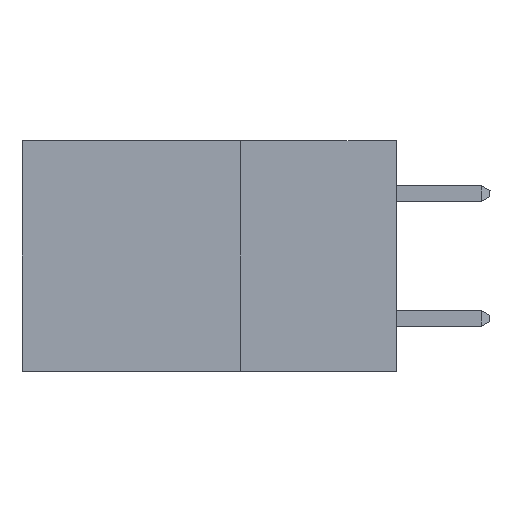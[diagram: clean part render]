
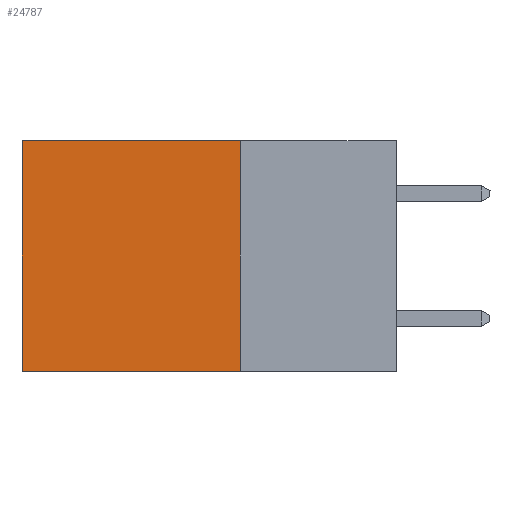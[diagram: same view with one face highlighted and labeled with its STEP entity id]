
A CAD part, left-side view. The second image highlights one B-rep face of the part: STEP entity #24787.
In plain terms, the highlighted planar face has unit normal (-1, 0, 0).
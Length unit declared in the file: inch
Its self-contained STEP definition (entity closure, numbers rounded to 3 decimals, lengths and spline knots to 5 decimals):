
#172 = CARTESIAN_POINT ( 'NONE',  ( 0.298, 0.6, 0. ) ) ;
#449 = VECTOR ( 'NONE', #8742, 39.37008 ) ;
#776 = LINE ( 'NONE', #6904, #15609 ) ;
#1443 = LINE ( 'NONE', #18984, #12046 ) ;
#1630 = ORIENTED_EDGE ( 'NONE', *, *, #18000, .F. ) ;
#1728 = EDGE_CURVE ( 'NONE', #15118, #23663, #1443, .T. ) ;
#1794 = CARTESIAN_POINT ( 'NONE',  ( 0.298, 0.25, -0.37 ) ) ;
#2021 = EDGE_CURVE ( 'NONE', #23663, #22549, #16575, .T. ) ;
#3612 = PLANE ( 'NONE',  #17691 ) ;
#5741 = DIRECTION ( 'NONE',  ( 0., 0., -1. ) ) ;
#6333 = ORIENTED_EDGE ( 'NONE', *, *, #1728, .T. ) ;
#6855 = CARTESIAN_POINT ( 'NONE',  ( 0.298, 0.25, -0.37 ) ) ;
#6904 = CARTESIAN_POINT ( 'NONE',  ( 0.298, 0.25, 0. ) ) ;
#8369 = VERTEX_POINT ( 'NONE', #6855 ) ;
#8742 = DIRECTION ( 'NONE',  ( 0., 0., -1. ) ) ;
#10619 = CARTESIAN_POINT ( 'NONE',  ( 0.298, 0.6, 0. ) ) ;
#12046 = VECTOR ( 'NONE', #21960, 39.37008 ) ;
#14359 = CARTESIAN_POINT ( 'NONE',  ( 0.298, 0.25, 0. ) ) ;
#15118 = VERTEX_POINT ( 'NONE', #14359 ) ;
#15148 = EDGE_CURVE ( 'NONE', #8369, #22549, #21484, .T. ) ;
#15527 = CARTESIAN_POINT ( 'NONE',  ( 0.298, 0.6, -0.37 ) ) ;
#15609 = VECTOR ( 'NONE', #25389, 39.37008 ) ;
#16119 = VECTOR ( 'NONE', #26548, 39.37008 ) ;
#16368 = EDGE_LOOP ( 'NONE', ( #20782, #21690, #1630, #6333 ) ) ;
#16575 = LINE ( 'NONE', #172, #449 ) ;
#17691 = AXIS2_PLACEMENT_3D ( 'NONE', #24203, #18217, #5741 ) ;
#18000 = EDGE_CURVE ( 'NONE', #15118, #8369, #776, .T. ) ;
#18217 = DIRECTION ( 'NONE',  ( 1., 0., 0. ) ) ;
#18984 = CARTESIAN_POINT ( 'NONE',  ( 0.298, 0.25, 0. ) ) ;
#20204 = FACE_OUTER_BOUND ( 'NONE', #16368, .T. ) ;
#20782 = ORIENTED_EDGE ( 'NONE', *, *, #2021, .T. ) ;
#21484 = LINE ( 'NONE', #1794, #16119 ) ;
#21690 = ORIENTED_EDGE ( 'NONE', *, *, #15148, .F. ) ;
#21960 = DIRECTION ( 'NONE',  ( 0., 1., 0. ) ) ;
#22549 = VERTEX_POINT ( 'NONE', #15527 ) ;
#23663 = VERTEX_POINT ( 'NONE', #10619 ) ;
#24203 = CARTESIAN_POINT ( 'NONE',  ( 0.298, 0.25, 0. ) ) ;
#24787 = ADVANCED_FACE ( 'NONE', ( #20204 ), #3612, .F. ) ;
#25389 = DIRECTION ( 'NONE',  ( 0., 0., -1. ) ) ;
#26548 = DIRECTION ( 'NONE',  ( 0., 1., 0. ) ) ;
